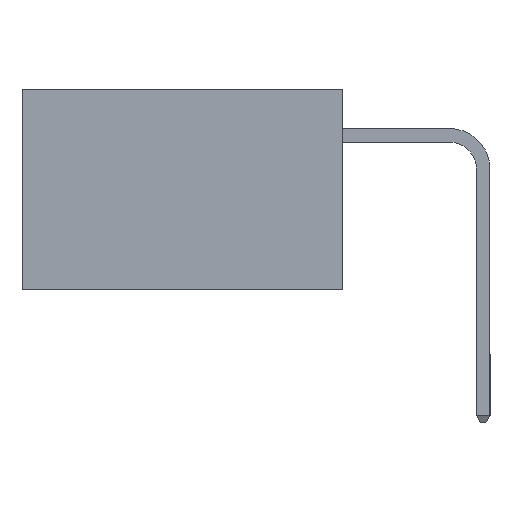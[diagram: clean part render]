
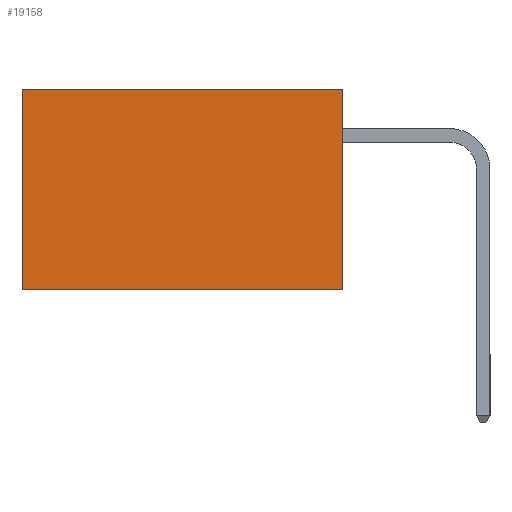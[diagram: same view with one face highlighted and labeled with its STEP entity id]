
A CAD part, left-side view. The second image highlights one B-rep face of the part: STEP entity #19158.
In plain terms, the highlighted planar face has unit normal (-1, 0, 0).
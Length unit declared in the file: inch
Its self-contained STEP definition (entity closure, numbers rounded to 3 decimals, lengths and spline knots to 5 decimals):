
#132 = DIRECTION ( 'NONE',  ( 0., 0., -1. ) ) ;
#691 = EDGE_LOOP ( 'NONE', ( #14409, #19063, #23610, #21045 ) ) ;
#1108 = LINE ( 'NONE', #3912, #24102 ) ;
#2753 = CARTESIAN_POINT ( 'NONE',  ( 0.277, 0.59, 0. ) ) ;
#2769 = EDGE_CURVE ( 'NONE', #8696, #26429, #17696, .T. ) ;
#3912 = CARTESIAN_POINT ( 'NONE',  ( 0.277, 0., 0. ) ) ;
#4002 = CARTESIAN_POINT ( 'NONE',  ( 0.277, 0.59, -0.37 ) ) ;
#6224 = VERTEX_POINT ( 'NONE', #2753 ) ;
#7195 = VECTOR ( 'NONE', #28627, 39.37008 ) ;
#7319 = AXIS2_PLACEMENT_3D ( 'NONE', #23077, #9835, #25296 ) ;
#7690 = CARTESIAN_POINT ( 'NONE',  ( 0.277, 0., -0.37 ) ) ;
#8696 = VERTEX_POINT ( 'NONE', #7690 ) ;
#9835 = DIRECTION ( 'NONE',  ( 1., 0., 0. ) ) ;
#13741 = EDGE_CURVE ( 'NONE', #23428, #6224, #1108, .T. ) ;
#14409 = ORIENTED_EDGE ( 'NONE', *, *, #24114, .T. ) ;
#14540 = CARTESIAN_POINT ( 'NONE',  ( 0.277, 0., -0.37 ) ) ;
#15384 = VECTOR ( 'NONE', #132, 39.37008 ) ;
#17624 = VECTOR ( 'NONE', #19073, 39.37008 ) ;
#17696 = LINE ( 'NONE', #22050, #7195 ) ;
#18705 = PLANE ( 'NONE',  #7319 ) ;
#19063 = ORIENTED_EDGE ( 'NONE', *, *, #2769, .F. ) ;
#19073 = DIRECTION ( 'NONE',  ( 0., 0., -1. ) ) ;
#19158 = ADVANCED_FACE ( 'NONE', ( #22357 ), #18705, .F. ) ;
#19766 = CARTESIAN_POINT ( 'NONE',  ( 0.277, 0., 0. ) ) ;
#21045 = ORIENTED_EDGE ( 'NONE', *, *, #13741, .T. ) ;
#22050 = CARTESIAN_POINT ( 'NONE',  ( 0.277, 0., -0.37 ) ) ;
#22319 = EDGE_CURVE ( 'NONE', #23428, #8696, #23462, .T. ) ;
#22357 = FACE_OUTER_BOUND ( 'NONE', #691, .T. ) ;
#23077 = CARTESIAN_POINT ( 'NONE',  ( 0.277, 0., -0.37 ) ) ;
#23428 = VERTEX_POINT ( 'NONE', #19766 ) ;
#23462 = LINE ( 'NONE', #14540, #17624 ) ;
#23610 = ORIENTED_EDGE ( 'NONE', *, *, #22319, .F. ) ;
#23924 = DIRECTION ( 'NONE',  ( 0., 1., 0. ) ) ;
#24102 = VECTOR ( 'NONE', #23924, 39.37008 ) ;
#24114 = EDGE_CURVE ( 'NONE', #6224, #26429, #27757, .T. ) ;
#25296 = DIRECTION ( 'NONE',  ( 0., 0., -1. ) ) ;
#26429 = VERTEX_POINT ( 'NONE', #4002 ) ;
#26755 = CARTESIAN_POINT ( 'NONE',  ( 0.277, 0.59, -0.37 ) ) ;
#27757 = LINE ( 'NONE', #26755, #15384 ) ;
#28627 = DIRECTION ( 'NONE',  ( 0., 1., 0. ) ) ;
